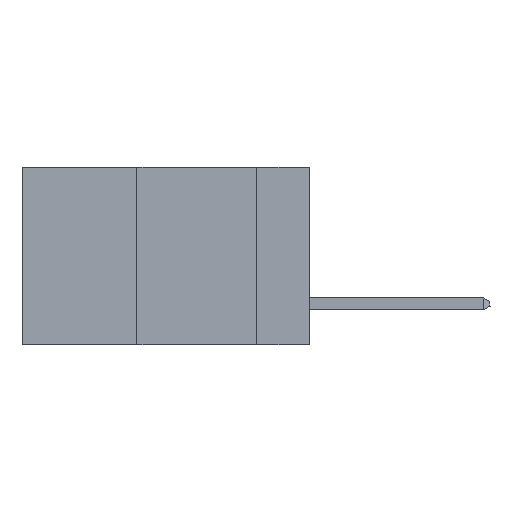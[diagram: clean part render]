
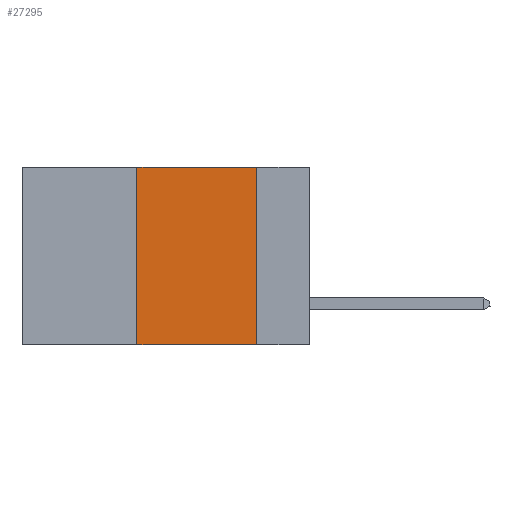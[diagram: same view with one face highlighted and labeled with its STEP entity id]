
A CAD part, left-side view. The second image highlights one B-rep face of the part: STEP entity #27295.
In plain terms, the highlighted planar face has unit normal (-1, 0, 0).
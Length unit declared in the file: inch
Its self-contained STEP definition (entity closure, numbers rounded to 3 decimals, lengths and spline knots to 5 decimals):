
#1488 = DIRECTION ( 'NONE',  ( 0., 0., -1. ) ) ;
#1502 = ORIENTED_EDGE ( 'NONE', *, *, #6139, .T. ) ;
#1741 = VECTOR ( 'NONE', #25770, 39.37008 ) ;
#1779 = DIRECTION ( 'NONE',  ( 0., 0., 1. ) ) ;
#2519 = ORIENTED_EDGE ( 'NONE', *, *, #19946, .F. ) ;
#2556 = VERTEX_POINT ( 'NONE', #26413 ) ;
#3310 = EDGE_LOOP ( 'NONE', ( #23637, #8692, #2519, #1502 ) ) ;
#3889 = LINE ( 'NONE', #10249, #28449 ) ;
#6046 = VERTEX_POINT ( 'NONE', #7866 ) ;
#6139 = EDGE_CURVE ( 'NONE', #2556, #6046, #24605, .T. ) ;
#6854 = FACE_OUTER_BOUND ( 'NONE', #3310, .T. ) ;
#7866 = CARTESIAN_POINT ( 'NONE',  ( 0., 0.11, -0.37 ) ) ;
#8692 = ORIENTED_EDGE ( 'NONE', *, *, #27377, .F. ) ;
#8833 = VECTOR ( 'NONE', #1779, 39.37008 ) ;
#9548 = LINE ( 'NONE', #10544, #8833 ) ;
#10249 = CARTESIAN_POINT ( 'NONE',  ( 0., 0.11, 0. ) ) ;
#10544 = CARTESIAN_POINT ( 'NONE',  ( 0., 0.36, 0. ) ) ;
#10994 = PLANE ( 'NONE',  #12330 ) ;
#12330 = AXIS2_PLACEMENT_3D ( 'NONE', #24957, #14969, #23698 ) ;
#13761 = LINE ( 'NONE', #14527, #27636 ) ;
#14527 = CARTESIAN_POINT ( 'NONE',  ( 0., 0.6, 0. ) ) ;
#14969 = DIRECTION ( 'NONE',  ( 1., 0., 0. ) ) ;
#17067 = CARTESIAN_POINT ( 'NONE',  ( 0., 0.6, -0.37 ) ) ;
#19519 = VERTEX_POINT ( 'NONE', #27147 ) ;
#19946 = EDGE_CURVE ( 'NONE', #2556, #19519, #9548, .T. ) ;
#21510 = VERTEX_POINT ( 'NONE', #23558 ) ;
#23453 = DIRECTION ( 'NONE',  ( 0., -1., 0. ) ) ;
#23558 = CARTESIAN_POINT ( 'NONE',  ( 0., 0.11, 0. ) ) ;
#23637 = ORIENTED_EDGE ( 'NONE', *, *, #25094, .F. ) ;
#23698 = DIRECTION ( 'NONE',  ( 0., 0., -1. ) ) ;
#24605 = LINE ( 'NONE', #17067, #1741 ) ;
#24957 = CARTESIAN_POINT ( 'NONE',  ( 0., 0.6, 0. ) ) ;
#25094 = EDGE_CURVE ( 'NONE', #21510, #6046, #3889, .T. ) ;
#25770 = DIRECTION ( 'NONE',  ( 0., -1., 0. ) ) ;
#26413 = CARTESIAN_POINT ( 'NONE',  ( 0., 0.36, -0.37 ) ) ;
#27147 = CARTESIAN_POINT ( 'NONE',  ( 0., 0.36, 0. ) ) ;
#27295 = ADVANCED_FACE ( 'NONE', ( #6854 ), #10994, .F. ) ;
#27377 = EDGE_CURVE ( 'NONE', #19519, #21510, #13761, .T. ) ;
#27636 = VECTOR ( 'NONE', #23453, 39.37008 ) ;
#28449 = VECTOR ( 'NONE', #1488, 39.37008 ) ;
